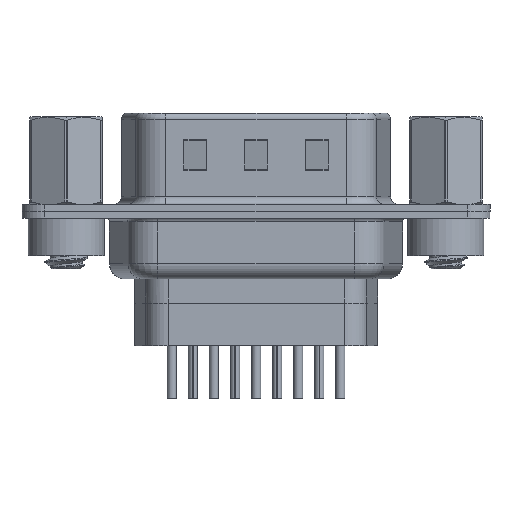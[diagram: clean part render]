
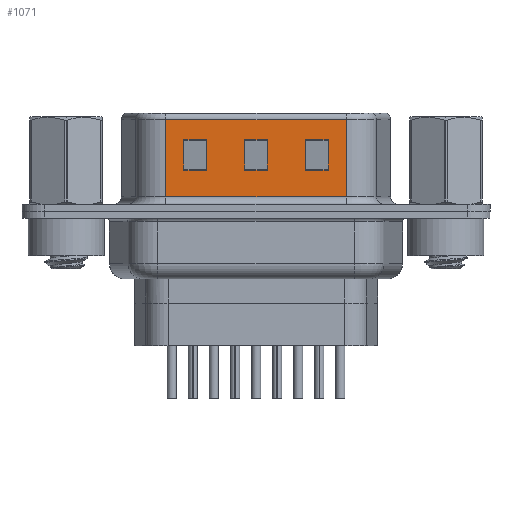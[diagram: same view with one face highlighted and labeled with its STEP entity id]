
A CAD part, front view. The second image highlights one B-rep face of the part: STEP entity #1071.
In plain terms, the highlighted planar face has unit normal (0, -1, 0).
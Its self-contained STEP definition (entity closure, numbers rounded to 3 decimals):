
#210 = DIRECTION ( 'NONE',  ( 1., 0., 0. ) ) ;
#386 = DIRECTION ( 'NONE',  ( 0., 0., 1. ) ) ;
#440 = FACE_BOUND ( 'NONE', #12836, .T. ) ;
#1071 = ADVANCED_FACE ( 'NONE', ( #440, #4569, #11959, #18864 ), #2616, .F. ) ;
#1124 = DIRECTION ( 'NONE',  ( 0., 0., 1. ) ) ;
#1532 = DIRECTION ( 'NONE',  ( 0., 0., 1. ) ) ;
#1598 = VECTOR ( 'NONE', #16861, 1000. ) ;
#2153 = LINE ( 'NONE', #16603, #10138 ) ;
#2416 = EDGE_CURVE ( 'NONE', #15221, #10371, #11162, .T. ) ;
#2559 = VERTEX_POINT ( 'NONE', #9700 ) ;
#2616 = PLANE ( 'NONE',  #17555 ) ;
#2689 = LINE ( 'NONE', #8290, #3961 ) ;
#2710 = VECTOR ( 'NONE', #386, 1000. ) ;
#2893 = DIRECTION ( 'NONE',  ( 0., 0., -1. ) ) ;
#3057 = ORIENTED_EDGE ( 'NONE', *, *, #8790, .F. ) ;
#3668 = EDGE_CURVE ( 'NONE', #10371, #10243, #10510, .T. ) ;
#3742 = EDGE_CURVE ( 'NONE', #19048, #15221, #6990, .T. ) ;
#3760 = CARTESIAN_POINT ( 'NONE',  ( 11.745, -4.58, 2.705 ) ) ;
#3921 = VECTOR ( 'NONE', #1124, 1000. ) ;
#3961 = VECTOR ( 'NONE', #8171, 1000. ) ;
#4196 = VERTEX_POINT ( 'NONE', #18472 ) ;
#4569 = FACE_BOUND ( 'NONE', #21178, .T. ) ;
#4954 = LINE ( 'NONE', #8351, #21951 ) ;
#5229 = VECTOR ( 'NONE', #18260, 1000. ) ;
#5748 = LINE ( 'NONE', #16656, #2710 ) ;
#6176 = EDGE_CURVE ( 'NONE', #15049, #20224, #6534, .T. ) ;
#6437 = EDGE_LOOP ( 'NONE', ( #19164, #17263, #9077, #17798 ) ) ;
#6534 = LINE ( 'NONE', #17688, #9061 ) ;
#6546 = VECTOR ( 'NONE', #1532, 1000. ) ;
#6639 = DIRECTION ( 'NONE',  ( -1., 0., 0. ) ) ;
#6951 = EDGE_CURVE ( 'NONE', #11419, #2559, #5748, .T. ) ;
#6990 = LINE ( 'NONE', #8824, #5229 ) ;
#7054 = VERTEX_POINT ( 'NONE', #15422 ) ;
#7778 = DIRECTION ( 'NONE',  ( 1., 0., 0. ) ) ;
#7944 = ORIENTED_EDGE ( 'NONE', *, *, #16191, .T. ) ;
#8171 = DIRECTION ( 'NONE',  ( 0., 0., -1. ) ) ;
#8219 = DIRECTION ( 'NONE',  ( 0., 1., 0. ) ) ;
#8270 = ORIENTED_EDGE ( 'NONE', *, *, #14898, .T. ) ;
#8290 = CARTESIAN_POINT ( 'NONE',  ( 18.445, -4.58, 6.52 ) ) ;
#8324 = VERTEX_POINT ( 'NONE', #18442 ) ;
#8351 = CARTESIAN_POINT ( 'NONE',  ( 14.445, -4.58, 2.705 ) ) ;
#8430 = EDGE_CURVE ( 'NONE', #17084, #15049, #14915, .T. ) ;
#8790 = EDGE_CURVE ( 'NONE', #17084, #9663, #2689, .T. ) ;
#8824 = CARTESIAN_POINT ( 'NONE',  ( 13.245, -4.58, 6.52 ) ) ;
#8893 = DIRECTION ( 'NONE',  ( 1., 0., 0. ) ) ;
#9061 = VECTOR ( 'NONE', #2893, 1000. ) ;
#9077 = ORIENTED_EDGE ( 'NONE', *, *, #2416, .T. ) ;
#9079 = EDGE_CURVE ( 'NONE', #8324, #16216, #18903, .T. ) ;
#9151 = VERTEX_POINT ( 'NONE', #20857 ) ;
#9656 = EDGE_CURVE ( 'NONE', #10243, #19048, #2153, .T. ) ;
#9662 = CARTESIAN_POINT ( 'NONE',  ( 18.445, -4.58, 0.95 ) ) ;
#9663 = VERTEX_POINT ( 'NONE', #14773 ) ;
#9700 = CARTESIAN_POINT ( 'NONE',  ( 15.745, -4.58, 4.705 ) ) ;
#9738 = CARTESIAN_POINT ( 'NONE',  ( 17.245, -4.58, 6.52 ) ) ;
#9882 = LINE ( 'NONE', #15213, #19368 ) ;
#10077 = ORIENTED_EDGE ( 'NONE', *, *, #19736, .T. ) ;
#10138 = VECTOR ( 'NONE', #210, 1000. ) ;
#10243 = VERTEX_POINT ( 'NONE', #23786 ) ;
#10371 = VERTEX_POINT ( 'NONE', #3760 ) ;
#10380 = CARTESIAN_POINT ( 'NONE',  ( 15.745, -4.58, 2.705 ) ) ;
#10510 = LINE ( 'NONE', #18141, #6546 ) ;
#11162 = LINE ( 'NONE', #12984, #11190 ) ;
#11190 = VECTOR ( 'NONE', #18550, 1000. ) ;
#11384 = CARTESIAN_POINT ( 'NONE',  ( 13.245, -4.58, 4.705 ) ) ;
#11419 = VERTEX_POINT ( 'NONE', #10380 ) ;
#11588 = EDGE_CURVE ( 'NONE', #16216, #7054, #9882, .T. ) ;
#11804 = CARTESIAN_POINT ( 'NONE',  ( 18.445, -4.58, 6.02 ) ) ;
#11959 = FACE_BOUND ( 'NONE', #6437, .T. ) ;
#12197 = EDGE_CURVE ( 'NONE', #15198, #4196, #15062, .T. ) ;
#12400 = EDGE_LOOP ( 'NONE', ( #3057, #14715, #18693, #8270 ) ) ;
#12773 = ORIENTED_EDGE ( 'NONE', *, *, #22387, .T. ) ;
#12836 = EDGE_LOOP ( 'NONE', ( #14035, #7944, #10077, #23466 ) ) ;
#12984 = CARTESIAN_POINT ( 'NONE',  ( 18.445, -4.58, 2.705 ) ) ;
#13039 = DIRECTION ( 'NONE',  ( 0., 0., -1. ) ) ;
#13337 = CARTESIAN_POINT ( 'NONE',  ( 14.445, -4.58, 4.705 ) ) ;
#13926 = CARTESIAN_POINT ( 'NONE',  ( 13.245, -4.58, 2.705 ) ) ;
#14035 = ORIENTED_EDGE ( 'NONE', *, *, #11588, .T. ) ;
#14715 = ORIENTED_EDGE ( 'NONE', *, *, #8430, .T. ) ;
#14773 = CARTESIAN_POINT ( 'NONE',  ( 18.445, -4.58, 0.95 ) ) ;
#14785 = ORIENTED_EDGE ( 'NONE', *, *, #12197, .T. ) ;
#14898 = EDGE_CURVE ( 'NONE', #20224, #9663, #22761, .T. ) ;
#14915 = LINE ( 'NONE', #22439, #1598 ) ;
#15049 = VERTEX_POINT ( 'NONE', #16276 ) ;
#15062 = LINE ( 'NONE', #9738, #18992 ) ;
#15111 = DIRECTION ( 'NONE',  ( 1., 0., 0. ) ) ;
#15198 = VERTEX_POINT ( 'NONE', #19156 ) ;
#15213 = CARTESIAN_POINT ( 'NONE',  ( 9.245, -4.58, 6.52 ) ) ;
#15221 = VERTEX_POINT ( 'NONE', #13926 ) ;
#15236 = CARTESIAN_POINT ( 'NONE',  ( 18.445, -4.58, 6.52 ) ) ;
#15322 = ORIENTED_EDGE ( 'NONE', *, *, #15398, .T. ) ;
#15398 = EDGE_CURVE ( 'NONE', #2559, #15198, #20155, .T. ) ;
#15422 = CARTESIAN_POINT ( 'NONE',  ( 9.245, -4.58, 2.705 ) ) ;
#15921 = DIRECTION ( 'NONE',  ( -1., 0., 0. ) ) ;
#16191 = EDGE_CURVE ( 'NONE', #7054, #9151, #4954, .T. ) ;
#16216 = VERTEX_POINT ( 'NONE', #21076 ) ;
#16276 = CARTESIAN_POINT ( 'NONE',  ( 6.545, -4.58, 6.02 ) ) ;
#16603 = CARTESIAN_POINT ( 'NONE',  ( 18.445, -4.58, 4.705 ) ) ;
#16656 = CARTESIAN_POINT ( 'NONE',  ( 15.745, -4.58, 6.52 ) ) ;
#16738 = CARTESIAN_POINT ( 'NONE',  ( 6.545, -4.58, 0.95 ) ) ;
#16861 = DIRECTION ( 'NONE',  ( -1., 0., 0. ) ) ;
#17084 = VERTEX_POINT ( 'NONE', #11804 ) ;
#17258 = VECTOR ( 'NONE', #15921, 1000. ) ;
#17263 = ORIENTED_EDGE ( 'NONE', *, *, #3742, .T. ) ;
#17555 = AXIS2_PLACEMENT_3D ( 'NONE', #15236, #8219, #20813 ) ;
#17617 = LINE ( 'NONE', #19786, #17258 ) ;
#17688 = CARTESIAN_POINT ( 'NONE',  ( 6.545, -4.58, 6.52 ) ) ;
#17798 = ORIENTED_EDGE ( 'NONE', *, *, #3668, .T. ) ;
#18141 = CARTESIAN_POINT ( 'NONE',  ( 11.745, -4.58, 6.52 ) ) ;
#18260 = DIRECTION ( 'NONE',  ( 0., 0., -1. ) ) ;
#18442 = CARTESIAN_POINT ( 'NONE',  ( 7.745, -4.58, 4.705 ) ) ;
#18451 = CARTESIAN_POINT ( 'NONE',  ( 22.445, -4.58, 4.705 ) ) ;
#18472 = CARTESIAN_POINT ( 'NONE',  ( 17.245, -4.58, 2.705 ) ) ;
#18550 = DIRECTION ( 'NONE',  ( -1., 0., 0. ) ) ;
#18693 = ORIENTED_EDGE ( 'NONE', *, *, #6176, .T. ) ;
#18864 = FACE_OUTER_BOUND ( 'NONE', #12400, .T. ) ;
#18903 = LINE ( 'NONE', #13337, #21403 ) ;
#18992 = VECTOR ( 'NONE', #22601, 1000. ) ;
#19048 = VERTEX_POINT ( 'NONE', #11384 ) ;
#19156 = CARTESIAN_POINT ( 'NONE',  ( 17.245, -4.58, 4.705 ) ) ;
#19164 = ORIENTED_EDGE ( 'NONE', *, *, #9656, .T. ) ;
#19222 = VECTOR ( 'NONE', #8893, 1000. ) ;
#19368 = VECTOR ( 'NONE', #13039, 1000. ) ;
#19736 = EDGE_CURVE ( 'NONE', #9151, #8324, #23201, .T. ) ;
#19786 = CARTESIAN_POINT ( 'NONE',  ( 22.445, -4.58, 2.705 ) ) ;
#20020 = VECTOR ( 'NONE', #15111, 1000. ) ;
#20155 = LINE ( 'NONE', #18451, #19222 ) ;
#20224 = VERTEX_POINT ( 'NONE', #16738 ) ;
#20813 = DIRECTION ( 'NONE',  ( 0., 0., 1. ) ) ;
#20857 = CARTESIAN_POINT ( 'NONE',  ( 7.745, -4.58, 2.705 ) ) ;
#21076 = CARTESIAN_POINT ( 'NONE',  ( 9.245, -4.58, 4.705 ) ) ;
#21178 = EDGE_LOOP ( 'NONE', ( #14785, #12773, #22734, #15322 ) ) ;
#21403 = VECTOR ( 'NONE', #7778, 1000. ) ;
#21951 = VECTOR ( 'NONE', #6639, 1000. ) ;
#22387 = EDGE_CURVE ( 'NONE', #4196, #11419, #17617, .T. ) ;
#22439 = CARTESIAN_POINT ( 'NONE',  ( 18.445, -4.58, 6.02 ) ) ;
#22601 = DIRECTION ( 'NONE',  ( 0., 0., -1. ) ) ;
#22734 = ORIENTED_EDGE ( 'NONE', *, *, #6951, .T. ) ;
#22761 = LINE ( 'NONE', #9662, #20020 ) ;
#23201 = LINE ( 'NONE', #23451, #3921 ) ;
#23451 = CARTESIAN_POINT ( 'NONE',  ( 7.745, -4.58, 6.52 ) ) ;
#23466 = ORIENTED_EDGE ( 'NONE', *, *, #9079, .T. ) ;
#23786 = CARTESIAN_POINT ( 'NONE',  ( 11.745, -4.58, 4.705 ) ) ;
